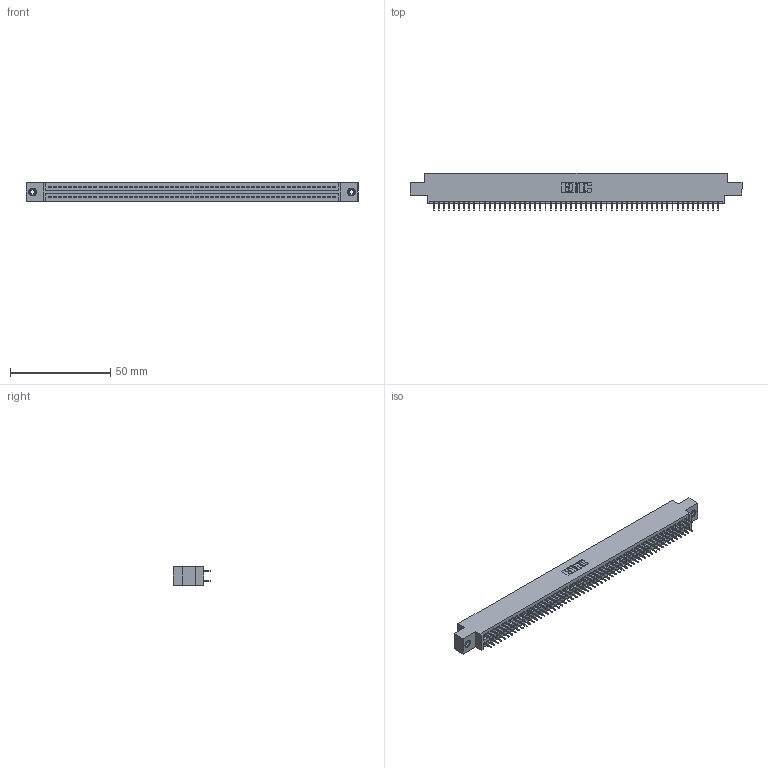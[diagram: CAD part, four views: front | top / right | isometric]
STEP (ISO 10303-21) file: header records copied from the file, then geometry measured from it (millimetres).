
FILE_DESCRIPTION (( 'STEP AP203' ), '1' );
FILE_NAME ('395-114-525-808.STEP', '2020-09-25T20:36:13', ( '' ), ( '' ), 'SwSTEP 2.0', 'SolidWorks 2020', '' );
FILE_SCHEMA (( 'CONFIG_CONTROL_DESIGN' ));
Length unit declared in the file: inch
Products named in the file (4): 345-292-001_345-293-125; 395-114-525-808; 345-250-001_345-250-003-102; 345 Part_0.170 Offset - 0.156 Dia-TI
Assembly tree (117 placements, depth 2):
  395-114-525-808
    345 Part_0.170 Offset - 0.156 Dia-TI
    345-292-001_345-293-125  x114
    345-250-001_345-250-003-102  x2
Bounding box: 165.99 x 18.72 x 9.4 mm (x, y, z)
Volume: 15956 mm3; surface area: 23467.7 mm2
Topology: 117 solids, 117 shells, 6346 faces, 17931 edges, 11490 vertices
Faces by surface type: plane 4562, cylinder 1768, cone 12, torus 4
Entity records: 44096 total; most frequent: CARTESIAN_POINT 7359, ORIENTED_EDGE 7286, DIRECTION 6497, EDGE_CURVE 3643, LINE 3267, VECTOR 3267, VERTEX_POINT 2420, AXIS2_PLACEMENT_3D 1615
